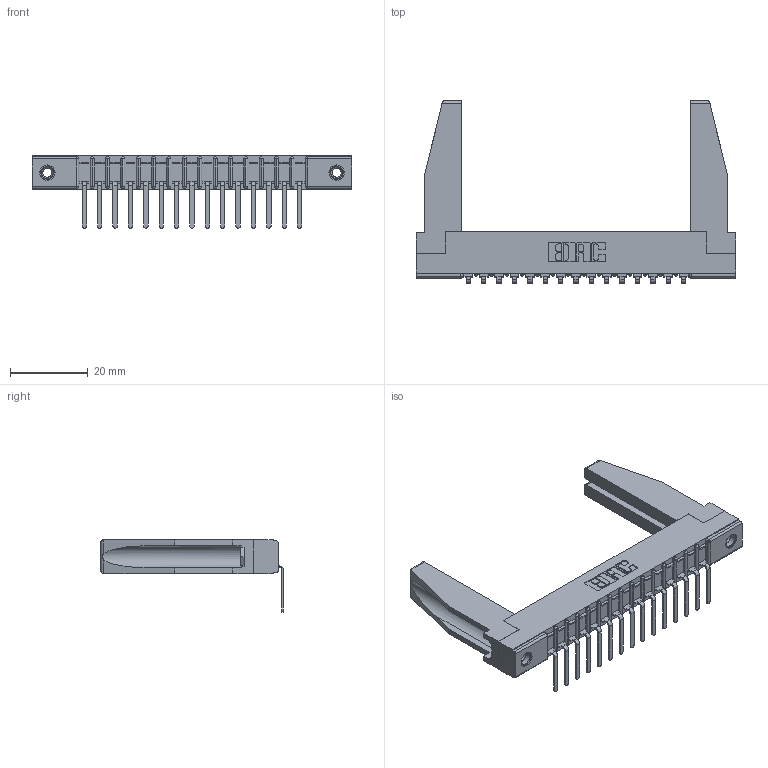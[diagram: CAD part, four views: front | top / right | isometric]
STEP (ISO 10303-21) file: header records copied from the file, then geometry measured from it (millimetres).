
FILE_DESCRIPTION (( 'STEP AP203' ), '1' );
FILE_NAME ('307-015-557-178.STEP', '2019-09-04T21:12:35', ( '' ), ( '' ), 'SwSTEP 2.0', 'SolidWorks 2016', '' );
FILE_SCHEMA (( 'CONFIG_CONTROL_DESIGN' ));
Length unit declared in the file: inch
Products named in the file (5): 307-220-078; 307 Part_.156 Dia Mounting Holes; 307-015-557-178; 345-250-001_345-250-001-102; 307-290-002_557
Assembly tree (20 placements, depth 2):
  307-015-557-178
    307 Part_.156 Dia Mounting Holes
    307-290-002_557  x15
    307-220-078  x2
    345-250-001_345-250-001-102  x2
Bounding box: 82.45 x 47.03 x 18.67 mm (x, y, z)
Volume: 9473.2 mm3; surface area: 13645.9 mm2
Topology: 20 solids, 20 shells, 1434 faces, 4313 edges, 2822 vertices
Faces by surface type: plane 859, cylinder 527, sphere 32, cone 12, torus 4
Entity records: 19481 total; most frequent: CARTESIAN_POINT 3282, ORIENTED_EDGE 3228, DIRECTION 3158, EDGE_CURVE 1614, LINE 1226, VECTOR 1226, VERTEX_POINT 1048, AXIS2_PLACEMENT_3D 966
